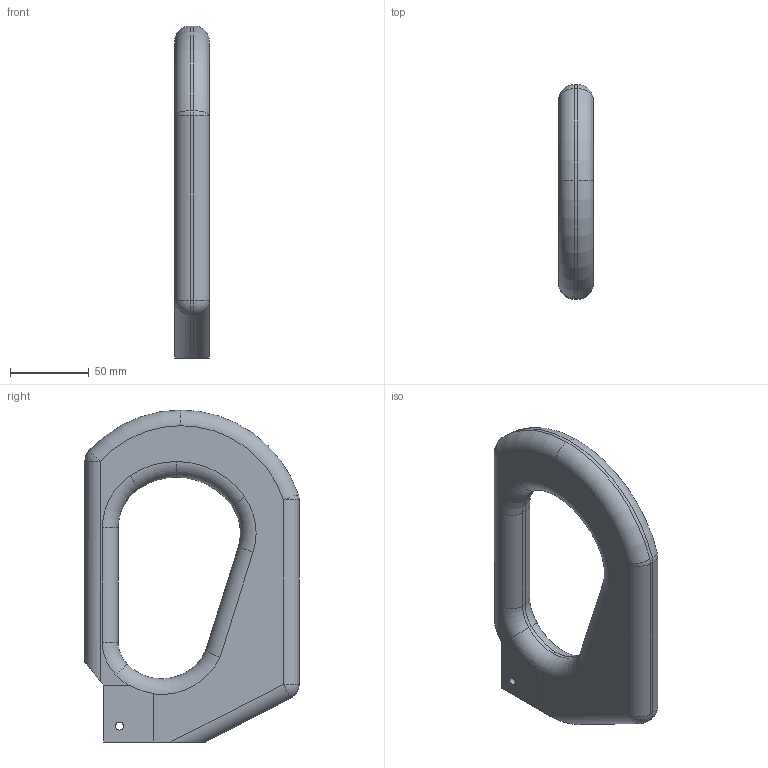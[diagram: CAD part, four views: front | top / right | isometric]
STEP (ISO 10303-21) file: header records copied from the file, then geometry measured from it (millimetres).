
FILE_DESCRIPTION (( 'STEP AP214' ), '1' );
FILE_NAME ('liberatorroundgrip.STEP', '2013-06-27T18:28:26', ( '' ), ( '' ), 'SwSTEP 2.0', 'SolidWorks 2012', '' );
FILE_SCHEMA (( 'AUTOMOTIVE_DESIGN' ));
Length unit declared in the file: millimetre
Products named in the file (1): liberatorroundgrip
Bounding box: 22.23 x 136.28 x 211.18 mm (x, y, z)
Volume: 353068 mm3; surface area: 50678.5 mm2
Topology: 1 solids, 1 shells, 66 faces, 168 edges, 97 vertices
Faces by surface type: cylinder 24, plane 20, torus 16, sphere 6
Entity records: 2038 total; most frequent: CARTESIAN_POINT 398, DIRECTION 366, ORIENTED_EDGE 324, EDGE_CURVE 162, AXIS2_PLACEMENT_3D 145, VERTEX_POINT 97, CIRCLE 78, VECTOR 76
